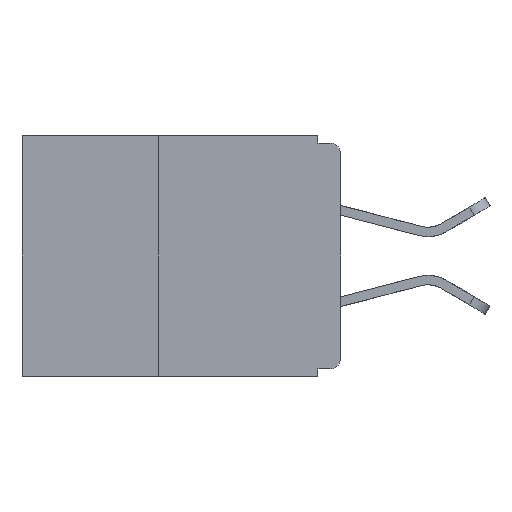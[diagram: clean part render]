
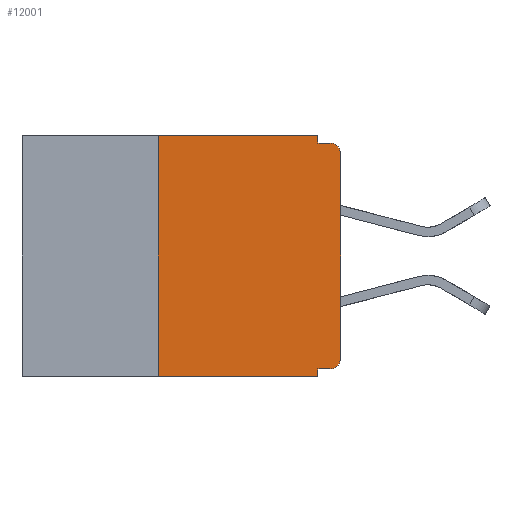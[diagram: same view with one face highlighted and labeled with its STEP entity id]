
A CAD part, left-side view. The second image highlights one B-rep face of the part: STEP entity #12001.
In plain terms, the highlighted planar face has unit normal (-1, 0, 0).
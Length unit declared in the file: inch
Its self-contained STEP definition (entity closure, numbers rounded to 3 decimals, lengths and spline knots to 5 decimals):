
#223 = ORIENTED_EDGE ( 'NONE', *, *, #9009, .F. ) ;
#226 = DIRECTION ( 'NONE',  ( 1., 0., 0. ) ) ;
#466 = CARTESIAN_POINT ( 'NONE',  ( 0., 0., -0.025 ) ) ;
#870 = ORIENTED_EDGE ( 'NONE', *, *, #12667, .T. ) ;
#927 = ORIENTED_EDGE ( 'NONE', *, *, #10501, .F. ) ;
#967 = DIRECTION ( 'NONE',  ( 0., 0., -1. ) ) ;
#1178 = CARTESIAN_POINT ( 'NONE',  ( 0., 0.031, 0. ) ) ;
#1563 = ORIENTED_EDGE ( 'NONE', *, *, #11571, .F. ) ;
#2368 = ORIENTED_EDGE ( 'NONE', *, *, #13039, .T. ) ;
#2395 = VERTEX_POINT ( 'NONE', #15731 ) ;
#2496 = EDGE_CURVE ( 'NONE', #10170, #14347, #11731, .T. ) ;
#2629 = EDGE_CURVE ( 'NONE', #14347, #9005, #13987, .T. ) ;
#2717 = VECTOR ( 'NONE', #14048, 39.37008 ) ;
#2846 = CARTESIAN_POINT ( 'NONE',  ( 0., 0.031, 0. ) ) ;
#2885 = VECTOR ( 'NONE', #19514, 39.37008 ) ;
#2987 = CARTESIAN_POINT ( 'NONE',  ( 0., 0.25, -0.33 ) ) ;
#3204 = CARTESIAN_POINT ( 'NONE',  ( 0., 0.031, -0.01 ) ) ;
#3402 = VERTEX_POINT ( 'NONE', #2846 ) ;
#3638 = AXIS2_PLACEMENT_3D ( 'NONE', #18248, #226, #11933 ) ;
#4006 = ORIENTED_EDGE ( 'NONE', *, *, #5218, .F. ) ;
#4151 = DIRECTION ( 'NONE',  ( 0., -1., 0. ) ) ;
#4697 = DIRECTION ( 'NONE',  ( 0., 0., 1. ) ) ;
#4764 = CARTESIAN_POINT ( 'NONE',  ( 0., 0.25, -0.33 ) ) ;
#5178 = DIRECTION ( 'NONE',  ( -1., 0., 0. ) ) ;
#5183 = CARTESIAN_POINT ( 'NONE',  ( 0., 0., -0.01 ) ) ;
#5218 = EDGE_CURVE ( 'NONE', #3402, #9969, #20081, .T. ) ;
#5248 = PLANE ( 'NONE',  #3638 ) ;
#5504 = CARTESIAN_POINT ( 'NONE',  ( 0., 0.031, -0.32 ) ) ;
#5623 = CARTESIAN_POINT ( 'NONE',  ( 0., 0.015, -0.025 ) ) ;
#6822 = DIRECTION ( 'NONE',  ( 0., -1., 0. ) ) ;
#7062 = ORIENTED_EDGE ( 'NONE', *, *, #8466, .F. ) ;
#7101 = CARTESIAN_POINT ( 'NONE',  ( 0., 0.015, -0.305 ) ) ;
#7674 = LINE ( 'NONE', #17142, #2717 ) ;
#7813 = VECTOR ( 'NONE', #19547, 39.37008 ) ;
#7985 = AXIS2_PLACEMENT_3D ( 'NONE', #7101, #18524, #8825 ) ;
#8013 = CARTESIAN_POINT ( 'NONE',  ( 0., 0.031, -0.33 ) ) ;
#8144 = DIRECTION ( 'NONE',  ( 0., 0., -1. ) ) ;
#8466 = EDGE_CURVE ( 'NONE', #13491, #3402, #17035, .T. ) ;
#8825 = DIRECTION ( 'NONE',  ( 0., 0., -1. ) ) ;
#9005 = VERTEX_POINT ( 'NONE', #12911 ) ;
#9009 = EDGE_CURVE ( 'NONE', #20522, #13491, #12422, .T. ) ;
#9638 = CARTESIAN_POINT ( 'NONE',  ( 0., 0.031, -0.33 ) ) ;
#9855 = VECTOR ( 'NONE', #11339, 39.37008 ) ;
#9912 = CARTESIAN_POINT ( 'NONE',  ( 0., 0.437, 0. ) ) ;
#9969 = VERTEX_POINT ( 'NONE', #3204 ) ;
#10080 = EDGE_CURVE ( 'NONE', #9969, #9005, #18451, .T. ) ;
#10170 = VERTEX_POINT ( 'NONE', #16859 ) ;
#10259 = VECTOR ( 'NONE', #4151, 39.37008 ) ;
#10403 = AXIS2_PLACEMENT_3D ( 'NONE', #5623, #5178, #8144 ) ;
#10501 = EDGE_CURVE ( 'NONE', #10808, #11803, #18435, .T. ) ;
#10808 = VERTEX_POINT ( 'NONE', #5504 ) ;
#11339 = DIRECTION ( 'NONE',  ( 0., 0., -1. ) ) ;
#11568 = FACE_OUTER_BOUND ( 'NONE', #14520, .T. ) ;
#11571 = EDGE_CURVE ( 'NONE', #2395, #10808, #7674, .T. ) ;
#11612 = CARTESIAN_POINT ( 'NONE',  ( 0., 0.25, 0. ) ) ;
#11731 = LINE ( 'NONE', #19483, #7813 ) ;
#11781 = CIRCLE ( 'NONE', #7985, 0.015 ) ;
#11803 = VERTEX_POINT ( 'NONE', #8013 ) ;
#11933 = DIRECTION ( 'NONE',  ( 0., 0., -1. ) ) ;
#12001 = ADVANCED_FACE ( 'NONE', ( #11568 ), #5248, .F. ) ;
#12404 = CARTESIAN_POINT ( 'NONE',  ( 0., 0.437, -0.33 ) ) ;
#12422 = LINE ( 'NONE', #2987, #16722 ) ;
#12667 = EDGE_CURVE ( 'NONE', #20522, #11803, #14569, .T. ) ;
#12911 = CARTESIAN_POINT ( 'NONE',  ( 0., 0.015, -0.01 ) ) ;
#13039 = EDGE_CURVE ( 'NONE', #2395, #10170, #11781, .T. ) ;
#13491 = VERTEX_POINT ( 'NONE', #11612 ) ;
#13987 = CIRCLE ( 'NONE', #10403, 0.015 ) ;
#14048 = DIRECTION ( 'NONE',  ( 0., 1., 0. ) ) ;
#14347 = VERTEX_POINT ( 'NONE', #466 ) ;
#14520 = EDGE_LOOP ( 'NONE', ( #16404, #17185, #18385, #4006, #7062, #223, #870, #927, #1563, #2368 ) ) ;
#14569 = LINE ( 'NONE', #12404, #10259 ) ;
#15731 = CARTESIAN_POINT ( 'NONE',  ( 0., 0.015, -0.32 ) ) ;
#15873 = VECTOR ( 'NONE', #967, 39.37008 ) ;
#16404 = ORIENTED_EDGE ( 'NONE', *, *, #2496, .T. ) ;
#16722 = VECTOR ( 'NONE', #4697, 39.37008 ) ;
#16859 = CARTESIAN_POINT ( 'NONE',  ( 0., 0., -0.305 ) ) ;
#17035 = LINE ( 'NONE', #9912, #2885 ) ;
#17142 = CARTESIAN_POINT ( 'NONE',  ( 0., 0., -0.32 ) ) ;
#17185 = ORIENTED_EDGE ( 'NONE', *, *, #2629, .T. ) ;
#18248 = CARTESIAN_POINT ( 'NONE',  ( 0., 0.437, 0. ) ) ;
#18385 = ORIENTED_EDGE ( 'NONE', *, *, #10080, .F. ) ;
#18435 = LINE ( 'NONE', #9638, #9855 ) ;
#18451 = LINE ( 'NONE', #5183, #18959 ) ;
#18524 = DIRECTION ( 'NONE',  ( -1., 0., 0. ) ) ;
#18959 = VECTOR ( 'NONE', #6822, 39.37008 ) ;
#19483 = CARTESIAN_POINT ( 'NONE',  ( 0., 0., 0. ) ) ;
#19514 = DIRECTION ( 'NONE',  ( 0., -1., 0. ) ) ;
#19547 = DIRECTION ( 'NONE',  ( 0., 0., 1. ) ) ;
#20081 = LINE ( 'NONE', #1178, #15873 ) ;
#20522 = VERTEX_POINT ( 'NONE', #4764 ) ;
